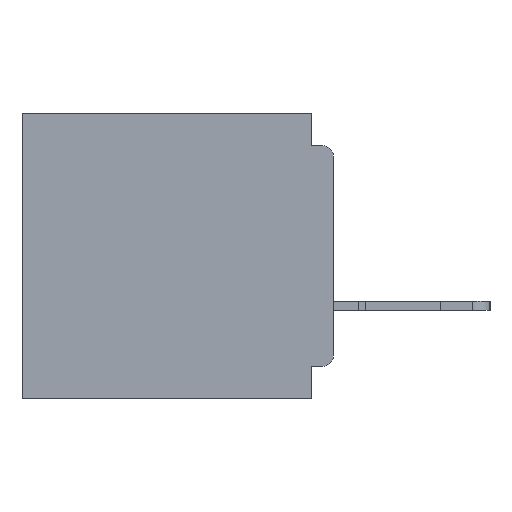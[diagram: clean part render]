
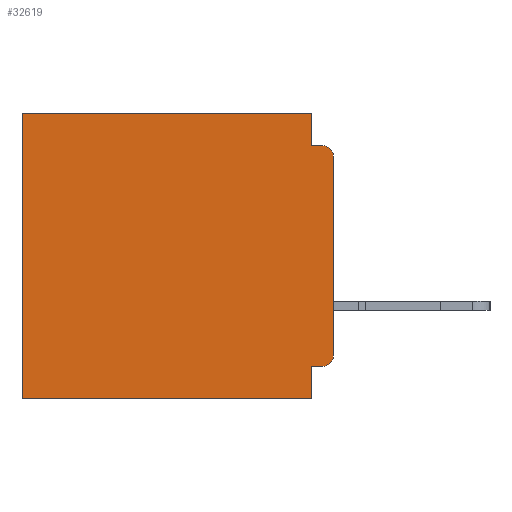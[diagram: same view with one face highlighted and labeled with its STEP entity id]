
A CAD part, left-side view. The second image highlights one B-rep face of the part: STEP entity #32619.
In plain terms, the highlighted planar face has unit normal (-1, 0, 0).
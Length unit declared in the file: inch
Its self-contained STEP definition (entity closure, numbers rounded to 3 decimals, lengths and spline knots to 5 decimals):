
#1042 = DIRECTION ( 'NONE',  ( 0., 0., -1. ) ) ;
#1050 = LINE ( 'NONE', #7315, #53604 ) ;
#1296 = VECTOR ( 'NONE', #1042, 39.37008 ) ;
#2482 = VECTOR ( 'NONE', #51518, 39.37008 ) ;
#2783 = EDGE_LOOP ( 'NONE', ( #4790, #65206, #20692, #31912, #25439, #38211, #9396, #3800, #63342, #25378 ) ) ;
#3800 = ORIENTED_EDGE ( 'NONE', *, *, #13321, .F. ) ;
#4092 = LINE ( 'NONE', #46469, #2482 ) ;
#4707 = VERTEX_POINT ( 'NONE', #18152 ) ;
#4790 = ORIENTED_EDGE ( 'NONE', *, *, #32931, .F. ) ;
#5657 = CARTESIAN_POINT ( 'NONE',  ( 0.3, 0.015, -0.06 ) ) ;
#5738 = EDGE_CURVE ( 'NONE', #31898, #39027, #1050, .T. ) ;
#6286 = LINE ( 'NONE', #45125, #31859 ) ;
#7315 = CARTESIAN_POINT ( 'NONE',  ( 0.3, 0., -0.4 ) ) ;
#7663 = DIRECTION ( 'NONE',  ( 0., 0., -1. ) ) ;
#8672 = AXIS2_PLACEMENT_3D ( 'NONE', #55516, #25117, #60539 ) ;
#8884 = VERTEX_POINT ( 'NONE', #30008 ) ;
#9396 = ORIENTED_EDGE ( 'NONE', *, *, #5738, .F. ) ;
#10757 = DIRECTION ( 'NONE',  ( 0., 0., -1. ) ) ;
#11278 = VECTOR ( 'NONE', #29170, 39.37008 ) ;
#13321 = EDGE_CURVE ( 'NONE', #36388, #31898, #19402, .T. ) ;
#16629 = CARTESIAN_POINT ( 'NONE',  ( 0.3, 0.031, 0. ) ) ;
#17219 = CIRCLE ( 'NONE', #27890, 0.015 ) ;
#18152 = CARTESIAN_POINT ( 'NONE',  ( 0.3, 0., -0.34 ) ) ;
#18305 = DIRECTION ( 'NONE',  ( -1., 0., 0. ) ) ;
#19402 = LINE ( 'NONE', #49242, #58292 ) ;
#20692 = ORIENTED_EDGE ( 'NONE', *, *, #61721, .F. ) ;
#22049 = CARTESIAN_POINT ( 'NONE',  ( 0.3, 0.015, -0.355 ) ) ;
#22402 = EDGE_CURVE ( 'NONE', #46731, #32010, #62811, .T. ) ;
#23872 = CARTESIAN_POINT ( 'NONE',  ( 0.3, 0.031, -0.4 ) ) ;
#24011 = CARTESIAN_POINT ( 'NONE',  ( 0.3, 0., -0.355 ) ) ;
#24464 = EDGE_CURVE ( 'NONE', #29923, #8884, #42015, .T. ) ;
#24684 = DIRECTION ( 'NONE',  ( 0., -1., 0. ) ) ;
#24904 = PLANE ( 'NONE',  #8672 ) ;
#25117 = DIRECTION ( 'NONE',  ( 1., 0., 0. ) ) ;
#25378 = ORIENTED_EDGE ( 'NONE', *, *, #30775, .T. ) ;
#25439 = ORIENTED_EDGE ( 'NONE', *, *, #55296, .T. ) ;
#25666 = CARTESIAN_POINT ( 'NONE',  ( 0.3, 0.437, 0. ) ) ;
#26146 = CARTESIAN_POINT ( 'NONE',  ( 0.3, 0.437, -0.4 ) ) ;
#27890 = AXIS2_PLACEMENT_3D ( 'NONE', #48766, #18305, #53847 ) ;
#29170 = DIRECTION ( 'NONE',  ( 0., 1., 0. ) ) ;
#29189 = EDGE_CURVE ( 'NONE', #65307, #39027, #33495, .T. ) ;
#29431 = VECTOR ( 'NONE', #7663, 39.37008 ) ;
#29923 = VERTEX_POINT ( 'NONE', #16629 ) ;
#30008 = CARTESIAN_POINT ( 'NONE',  ( 0.3, 0.031, -0.045 ) ) ;
#30775 = EDGE_CURVE ( 'NONE', #56490, #4707, #17219, .T. ) ;
#30955 = FACE_OUTER_BOUND ( 'NONE', #2783, .T. ) ;
#31859 = VECTOR ( 'NONE', #24684, 39.37008 ) ;
#31898 = VERTEX_POINT ( 'NONE', #23872 ) ;
#31912 = ORIENTED_EDGE ( 'NONE', *, *, #24464, .F. ) ;
#32010 = VERTEX_POINT ( 'NONE', #55147 ) ;
#32619 = ADVANCED_FACE ( 'NONE', ( #30955 ), #24904, .F. ) ;
#32931 = EDGE_CURVE ( 'NONE', #46731, #4707, #44508, .T. ) ;
#33495 = LINE ( 'NONE', #26146, #45375 ) ;
#36270 = CARTESIAN_POINT ( 'NONE',  ( 0.3, 0.437, -0.4 ) ) ;
#36388 = VERTEX_POINT ( 'NONE', #62557 ) ;
#36625 = EDGE_CURVE ( 'NONE', #56490, #36388, #40017, .T. ) ;
#38211 = ORIENTED_EDGE ( 'NONE', *, *, #29189, .T. ) ;
#38522 = CARTESIAN_POINT ( 'NONE',  ( 0.3, 0., -0.06 ) ) ;
#39027 = VERTEX_POINT ( 'NONE', #36270 ) ;
#40017 = LINE ( 'NONE', #24011, #11278 ) ;
#41338 = DIRECTION ( 'NONE',  ( -1., 0., 0. ) ) ;
#42015 = LINE ( 'NONE', #61931, #1296 ) ;
#44508 = LINE ( 'NONE', #48398, #29431 ) ;
#45125 = CARTESIAN_POINT ( 'NONE',  ( 0.3, 0., -0.045 ) ) ;
#45375 = VECTOR ( 'NONE', #51387, 39.37008 ) ;
#46469 = CARTESIAN_POINT ( 'NONE',  ( 0.3, 0., 0. ) ) ;
#46731 = VERTEX_POINT ( 'NONE', #38522 ) ;
#48398 = CARTESIAN_POINT ( 'NONE',  ( 0.3, 0., -0.4 ) ) ;
#48766 = CARTESIAN_POINT ( 'NONE',  ( 0.3, 0.015, -0.34 ) ) ;
#49242 = CARTESIAN_POINT ( 'NONE',  ( 0.3, 0.031, -0.4 ) ) ;
#49626 = AXIS2_PLACEMENT_3D ( 'NONE', #5657, #41338, #10757 ) ;
#51387 = DIRECTION ( 'NONE',  ( 0., 0., -1. ) ) ;
#51518 = DIRECTION ( 'NONE',  ( 0., 1., 0. ) ) ;
#53604 = VECTOR ( 'NONE', #58188, 39.37008 ) ;
#53847 = DIRECTION ( 'NONE',  ( 0., 0., -1. ) ) ;
#54323 = DIRECTION ( 'NONE',  ( 0., 0., -1. ) ) ;
#55147 = CARTESIAN_POINT ( 'NONE',  ( 0.3, 0.015, -0.045 ) ) ;
#55296 = EDGE_CURVE ( 'NONE', #29923, #65307, #4092, .T. ) ;
#55516 = CARTESIAN_POINT ( 'NONE',  ( 0.3, 0., -0.4 ) ) ;
#56490 = VERTEX_POINT ( 'NONE', #22049 ) ;
#58188 = DIRECTION ( 'NONE',  ( 0., 1., 0. ) ) ;
#58292 = VECTOR ( 'NONE', #54323, 39.37008 ) ;
#60539 = DIRECTION ( 'NONE',  ( 0., 0., -1. ) ) ;
#61721 = EDGE_CURVE ( 'NONE', #8884, #32010, #6286, .T. ) ;
#61931 = CARTESIAN_POINT ( 'NONE',  ( 0.3, 0.031, 0. ) ) ;
#62557 = CARTESIAN_POINT ( 'NONE',  ( 0.3, 0.031, -0.355 ) ) ;
#62811 = CIRCLE ( 'NONE', #49626, 0.015 ) ;
#63342 = ORIENTED_EDGE ( 'NONE', *, *, #36625, .F. ) ;
#65206 = ORIENTED_EDGE ( 'NONE', *, *, #22402, .T. ) ;
#65307 = VERTEX_POINT ( 'NONE', #25666 ) ;
